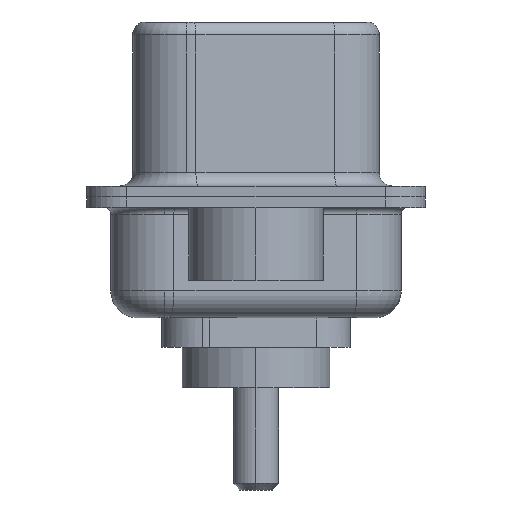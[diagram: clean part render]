
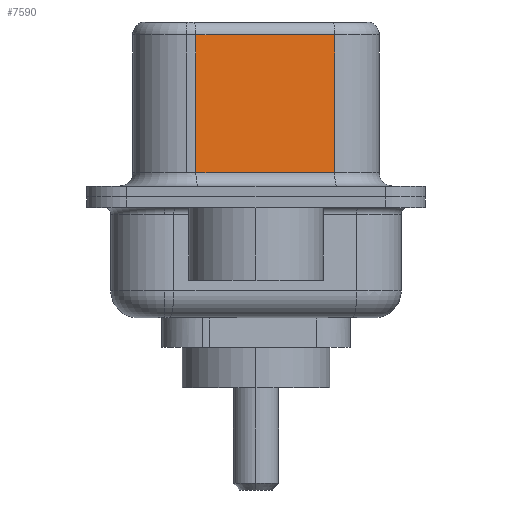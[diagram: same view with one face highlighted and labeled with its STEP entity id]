
A CAD part, left-side view. The second image highlights one B-rep face of the part: STEP entity #7590.
In plain terms, the highlighted planar face has unit normal (-0.985, -0.174, 0).
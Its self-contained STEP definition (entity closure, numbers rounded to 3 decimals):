
#1019 = FACE_OUTER_BOUND ( 'NONE', #9648, .T. ) ;
#1368 = VECTOR ( 'NONE', #10139, 1000. ) ;
#1623 = CARTESIAN_POINT ( 'NONE',  ( 4.565, -2.927, 6.52 ) ) ;
#1811 = ORIENTED_EDGE ( 'NONE', *, *, #15358, .T. ) ;
#2252 = CARTESIAN_POINT ( 'NONE',  ( 4.565, -2.927, 6.02 ) ) ;
#2620 = LINE ( 'NONE', #1623, #15119 ) ;
#2919 = DIRECTION ( 'NONE',  ( 0., 0., -1. ) ) ;
#3363 = CARTESIAN_POINT ( 'NONE',  ( 3.655, 2.233, 6.52 ) ) ;
#4574 = CARTESIAN_POINT ( 'NONE',  ( 4.565, -2.927, 0.9 ) ) ;
#5340 = AXIS2_PLACEMENT_3D ( 'NONE', #9093, #9965, #9186 ) ;
#5534 = VERTEX_POINT ( 'NONE', #8433 ) ;
#5671 = VECTOR ( 'NONE', #5945, 1000. ) ;
#5945 = DIRECTION ( 'NONE',  ( 0.174, -0.985, 0. ) ) ;
#6293 = ORIENTED_EDGE ( 'NONE', *, *, #9817, .F. ) ;
#6781 = VECTOR ( 'NONE', #2919, 1000. ) ;
#7075 = VERTEX_POINT ( 'NONE', #15425 ) ;
#7170 = DIRECTION ( 'NONE',  ( 0., 0., -1. ) ) ;
#7590 = ADVANCED_FACE ( 'NONE', ( #1019 ), #9922, .F. ) ;
#7869 = EDGE_CURVE ( 'NONE', #7075, #5534, #10038, .T. ) ;
#8433 = CARTESIAN_POINT ( 'NONE',  ( 3.655, 2.233, 0.9 ) ) ;
#8812 = VERTEX_POINT ( 'NONE', #10989 ) ;
#8950 = LINE ( 'NONE', #13174, #5671 ) ;
#9056 = EDGE_CURVE ( 'NONE', #8812, #7075, #10937, .T. ) ;
#9093 = CARTESIAN_POINT ( 'NONE',  ( 4.565, -2.927, 6.52 ) ) ;
#9186 = DIRECTION ( 'NONE',  ( -0.174, 0.985, 0. ) ) ;
#9648 = EDGE_LOOP ( 'NONE', ( #6293, #15392, #9750, #1811 ) ) ;
#9750 = ORIENTED_EDGE ( 'NONE', *, *, #7869, .T. ) ;
#9817 = EDGE_CURVE ( 'NONE', #8812, #11613, #2620, .T. ) ;
#9922 = PLANE ( 'NONE',  #5340 ) ;
#9965 = DIRECTION ( 'NONE',  ( 0.985, 0.174, 0. ) ) ;
#10038 = LINE ( 'NONE', #3363, #6781 ) ;
#10139 = DIRECTION ( 'NONE',  ( -0.174, 0.985, 0. ) ) ;
#10937 = LINE ( 'NONE', #2252, #1368 ) ;
#10989 = CARTESIAN_POINT ( 'NONE',  ( 4.565, -2.927, 6.02 ) ) ;
#11613 = VERTEX_POINT ( 'NONE', #4574 ) ;
#13174 = CARTESIAN_POINT ( 'NONE',  ( 4.565, -2.927, 0.9 ) ) ;
#15119 = VECTOR ( 'NONE', #7170, 1000. ) ;
#15358 = EDGE_CURVE ( 'NONE', #5534, #11613, #8950, .T. ) ;
#15392 = ORIENTED_EDGE ( 'NONE', *, *, #9056, .T. ) ;
#15425 = CARTESIAN_POINT ( 'NONE',  ( 3.655, 2.233, 6.02 ) ) ;
